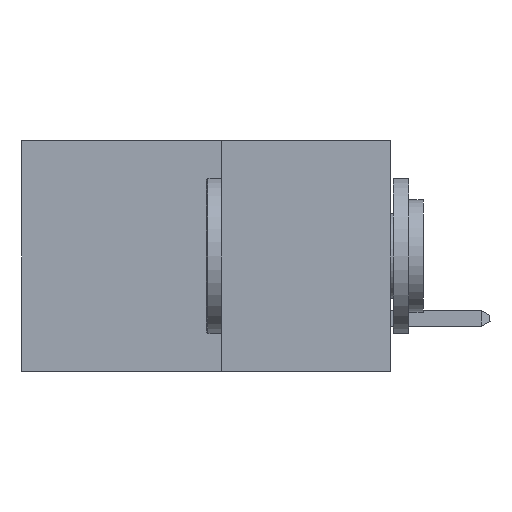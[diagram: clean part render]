
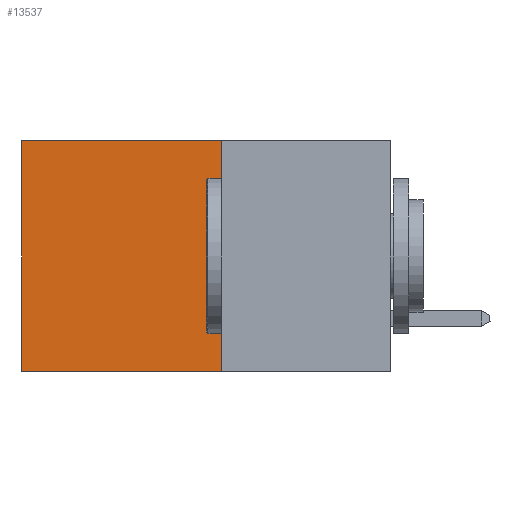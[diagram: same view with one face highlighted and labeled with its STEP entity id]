
A CAD part, left-side view. The second image highlights one B-rep face of the part: STEP entity #13537.
In plain terms, the highlighted planar face has unit normal (-1, 0, 0).
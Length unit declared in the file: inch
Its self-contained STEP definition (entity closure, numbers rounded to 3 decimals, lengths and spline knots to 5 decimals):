
#695 = ORIENTED_EDGE ( 'NONE', *, *, #13797, .F. ) ;
#1203 = VECTOR ( 'NONE', #8242, 39.37008 ) ;
#1547 = VERTEX_POINT ( 'NONE', #14786 ) ;
#2343 = EDGE_CURVE ( 'NONE', #3146, #12024, #5351, .T. ) ;
#2406 = EDGE_CURVE ( 'NONE', #3146, #4515, #15725, .T. ) ;
#2998 = CARTESIAN_POINT ( 'NONE',  ( 0.277, 0.59, 0. ) ) ;
#3146 = VERTEX_POINT ( 'NONE', #13814 ) ;
#3508 = LINE ( 'NONE', #14888, #11278 ) ;
#4343 = ORIENTED_EDGE ( 'NONE', *, *, #7733, .T. ) ;
#4515 = VERTEX_POINT ( 'NONE', #15494 ) ;
#4664 = DIRECTION ( 'NONE',  ( 0., 0., -1. ) ) ;
#5351 = LINE ( 'NONE', #5360, #1203 ) ;
#5360 = CARTESIAN_POINT ( 'NONE',  ( 0.277, 0.27, 0. ) ) ;
#6624 = PLANE ( 'NONE',  #15555 ) ;
#7733 = EDGE_CURVE ( 'NONE', #12024, #1547, #10462, .T. ) ;
#7912 = FACE_OUTER_BOUND ( 'NONE', #12383, .T. ) ;
#8200 = DIRECTION ( 'NONE',  ( 1., 0., 0. ) ) ;
#8242 = DIRECTION ( 'NONE',  ( 0., 1., 0. ) ) ;
#9682 = CARTESIAN_POINT ( 'NONE',  ( 0.277, 0.27, -0.37 ) ) ;
#10462 = LINE ( 'NONE', #12152, #14053 ) ;
#11278 = VECTOR ( 'NONE', #16442, 39.37008 ) ;
#11654 = VECTOR ( 'NONE', #4664, 39.37008 ) ;
#12024 = VERTEX_POINT ( 'NONE', #2998 ) ;
#12152 = CARTESIAN_POINT ( 'NONE',  ( 0.277, 0.59, -0.37 ) ) ;
#12383 = EDGE_LOOP ( 'NONE', ( #4343, #695, #18559, #15464 ) ) ;
#12900 = DIRECTION ( 'NONE',  ( 0., 0., -1. ) ) ;
#13537 = ADVANCED_FACE ( 'NONE', ( #7912 ), #6624, .F. ) ;
#13797 = EDGE_CURVE ( 'NONE', #4515, #1547, #3508, .T. ) ;
#13814 = CARTESIAN_POINT ( 'NONE',  ( 0.277, 0.27, 0. ) ) ;
#14053 = VECTOR ( 'NONE', #12900, 39.37008 ) ;
#14786 = CARTESIAN_POINT ( 'NONE',  ( 0.277, 0.59, -0.37 ) ) ;
#14888 = CARTESIAN_POINT ( 'NONE',  ( 0.277, 0.27, -0.37 ) ) ;
#15464 = ORIENTED_EDGE ( 'NONE', *, *, #2343, .T. ) ;
#15494 = CARTESIAN_POINT ( 'NONE',  ( 0.277, 0.27, -0.37 ) ) ;
#15555 = AXIS2_PLACEMENT_3D ( 'NONE', #9682, #8200, #18909 ) ;
#15725 = LINE ( 'NONE', #16936, #11654 ) ;
#16442 = DIRECTION ( 'NONE',  ( 0., 1., 0. ) ) ;
#16936 = CARTESIAN_POINT ( 'NONE',  ( 0.277, 0.27, -0.37 ) ) ;
#18559 = ORIENTED_EDGE ( 'NONE', *, *, #2406, .F. ) ;
#18909 = DIRECTION ( 'NONE',  ( 0., 0., -1. ) ) ;
